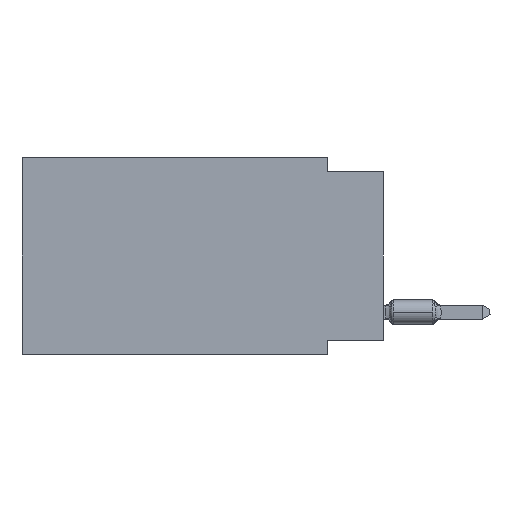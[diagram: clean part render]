
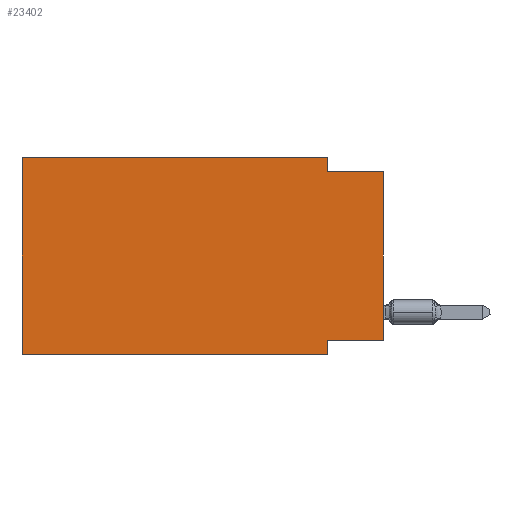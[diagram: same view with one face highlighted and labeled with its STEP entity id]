
A CAD part, left-side view. The second image highlights one B-rep face of the part: STEP entity #23402.
In plain terms, the highlighted planar face has unit normal (-1, 0, 0).
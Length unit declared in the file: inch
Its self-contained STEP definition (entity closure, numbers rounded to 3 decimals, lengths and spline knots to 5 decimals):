
#616 = CARTESIAN_POINT ( 'NONE',  ( 0., 0.645, 0. ) ) ;
#962 = EDGE_CURVE ( 'NONE', #14522, #18789, #14931, .T. ) ;
#1346 = LINE ( 'NONE', #12555, #16508 ) ;
#1754 = DIRECTION ( 'NONE',  ( 0., -1., 0. ) ) ;
#1875 = DIRECTION ( 'NONE',  ( 0., 0., -1. ) ) ;
#2001 = FACE_OUTER_BOUND ( 'NONE', #24177, .T. ) ;
#2039 = VECTOR ( 'NONE', #15341, 39.37008 ) ;
#2153 = CARTESIAN_POINT ( 'NONE',  ( 0., 0.1, -0.35 ) ) ;
#3067 = ORIENTED_EDGE ( 'NONE', *, *, #15340, .F. ) ;
#3164 = DIRECTION ( 'NONE',  ( 0., 0., -1. ) ) ;
#3292 = CARTESIAN_POINT ( 'NONE',  ( 0., 0.1, -0.35 ) ) ;
#3315 = ORIENTED_EDGE ( 'NONE', *, *, #20678, .T. ) ;
#3845 = EDGE_CURVE ( 'NONE', #17899, #18789, #5003, .T. ) ;
#3899 = VECTOR ( 'NONE', #6450, 39.37008 ) ;
#4285 = VERTEX_POINT ( 'NONE', #16670 ) ;
#4442 = CARTESIAN_POINT ( 'NONE',  ( 0., 0.1, -0.325 ) ) ;
#4597 = DIRECTION ( 'NONE',  ( 0., 0., -1. ) ) ;
#4785 = VECTOR ( 'NONE', #4597, 39.37008 ) ;
#5003 = LINE ( 'NONE', #3292, #20379 ) ;
#5019 = DIRECTION ( 'NONE',  ( 0., -1., 0. ) ) ;
#5180 = CARTESIAN_POINT ( 'NONE',  ( 0., 0., 0. ) ) ;
#5896 = VERTEX_POINT ( 'NONE', #24128 ) ;
#6450 = DIRECTION ( 'NONE',  ( 0., 1., 0. ) ) ;
#6769 = VECTOR ( 'NONE', #20432, 39.37008 ) ;
#7169 = ORIENTED_EDGE ( 'NONE', *, *, #20135, .F. ) ;
#7492 = EDGE_CURVE ( 'NONE', #12707, #18474, #1346, .T. ) ;
#7671 = CARTESIAN_POINT ( 'NONE',  ( 0., 0., -0.025 ) ) ;
#8169 = EDGE_CURVE ( 'NONE', #4285, #16189, #19013, .T. ) ;
#8278 = EDGE_CURVE ( 'NONE', #18474, #4285, #16049, .T. ) ;
#8428 = ORIENTED_EDGE ( 'NONE', *, *, #962, .T. ) ;
#8710 = VECTOR ( 'NONE', #12718, 39.37008 ) ;
#8889 = CARTESIAN_POINT ( 'NONE',  ( 0., 0., -0.325 ) ) ;
#9513 = PLANE ( 'NONE',  #10329 ) ;
#10329 = AXIS2_PLACEMENT_3D ( 'NONE', #17020, #15180, #1875 ) ;
#11221 = ORIENTED_EDGE ( 'NONE', *, *, #3845, .F. ) ;
#12109 = LINE ( 'NONE', #8889, #3899 ) ;
#12555 = CARTESIAN_POINT ( 'NONE',  ( 0., 0.645, 0. ) ) ;
#12707 = VERTEX_POINT ( 'NONE', #616 ) ;
#12718 = DIRECTION ( 'NONE',  ( 0., 0., 1. ) ) ;
#13195 = CARTESIAN_POINT ( 'NONE',  ( 0., 0.645, 0. ) ) ;
#13209 = CARTESIAN_POINT ( 'NONE',  ( 0., 0.645, -0.35 ) ) ;
#13438 = LINE ( 'NONE', #13195, #6769 ) ;
#13732 = CARTESIAN_POINT ( 'NONE',  ( 0., 0., -0.025 ) ) ;
#14522 = VERTEX_POINT ( 'NONE', #17164 ) ;
#14931 = LINE ( 'NONE', #13209, #21617 ) ;
#15180 = DIRECTION ( 'NONE',  ( 1., 0., 0. ) ) ;
#15340 = EDGE_CURVE ( 'NONE', #14522, #12707, #13438, .T. ) ;
#15341 = DIRECTION ( 'NONE',  ( 0., -1., 0. ) ) ;
#16049 = LINE ( 'NONE', #21815, #4785 ) ;
#16189 = VERTEX_POINT ( 'NONE', #7671 ) ;
#16194 = CARTESIAN_POINT ( 'NONE',  ( 0., 0.1, 0. ) ) ;
#16508 = VECTOR ( 'NONE', #5019, 39.37008 ) ;
#16670 = CARTESIAN_POINT ( 'NONE',  ( 0., 0.1, -0.025 ) ) ;
#17020 = CARTESIAN_POINT ( 'NONE',  ( 0., 0.645, 0. ) ) ;
#17164 = CARTESIAN_POINT ( 'NONE',  ( 0., 0.645, -0.35 ) ) ;
#17899 = VERTEX_POINT ( 'NONE', #4442 ) ;
#18474 = VERTEX_POINT ( 'NONE', #16194 ) ;
#18789 = VERTEX_POINT ( 'NONE', #2153 ) ;
#19013 = LINE ( 'NONE', #13732, #2039 ) ;
#19347 = ORIENTED_EDGE ( 'NONE', *, *, #8278, .F. ) ;
#20135 = EDGE_CURVE ( 'NONE', #5896, #17899, #12109, .T. ) ;
#20180 = ORIENTED_EDGE ( 'NONE', *, *, #8169, .F. ) ;
#20379 = VECTOR ( 'NONE', #3164, 39.37008 ) ;
#20432 = DIRECTION ( 'NONE',  ( 0., 0., 1. ) ) ;
#20678 = EDGE_CURVE ( 'NONE', #5896, #16189, #22013, .T. ) ;
#21617 = VECTOR ( 'NONE', #1754, 39.37008 ) ;
#21815 = CARTESIAN_POINT ( 'NONE',  ( 0., 0.1, 0. ) ) ;
#22013 = LINE ( 'NONE', #5180, #8710 ) ;
#23402 = ADVANCED_FACE ( 'NONE', ( #2001 ), #9513, .F. ) ;
#23935 = ORIENTED_EDGE ( 'NONE', *, *, #7492, .F. ) ;
#24128 = CARTESIAN_POINT ( 'NONE',  ( 0., 0., -0.325 ) ) ;
#24177 = EDGE_LOOP ( 'NONE', ( #3315, #20180, #19347, #23935, #3067, #8428, #11221, #7169 ) ) ;
